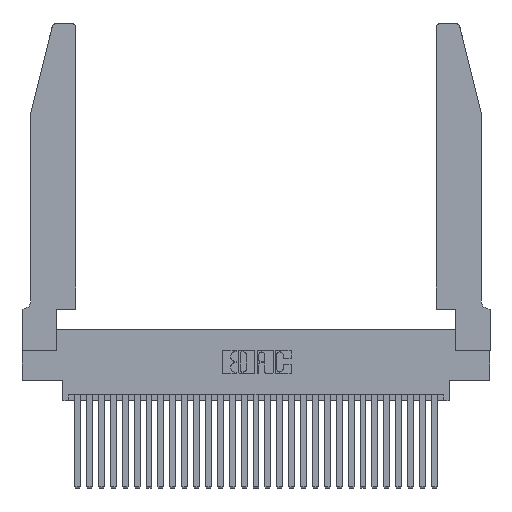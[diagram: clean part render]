
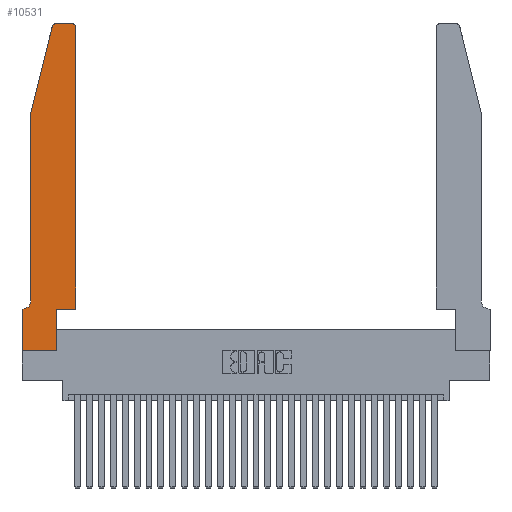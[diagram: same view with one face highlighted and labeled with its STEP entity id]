
A CAD part, top view. The second image highlights one B-rep face of the part: STEP entity #10531.
In plain terms, the highlighted planar face has unit normal (0, 0, 1).
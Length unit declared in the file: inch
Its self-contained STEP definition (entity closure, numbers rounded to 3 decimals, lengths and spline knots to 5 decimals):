
#665 = EDGE_CURVE ( 'NONE', #15499, #2017, #19378, .T. ) ;
#767 = AXIS2_PLACEMENT_3D ( 'NONE', #4609, #9463, #13971 ) ;
#970 = VECTOR ( 'NONE', #5539, 39.37008 ) ;
#1278 = LINE ( 'NONE', #6283, #6064 ) ;
#1909 = VERTEX_POINT ( 'NONE', #15012 ) ;
#2017 = VERTEX_POINT ( 'NONE', #3666 ) ;
#2301 = VERTEX_POINT ( 'NONE', #23953 ) ;
#2540 = LINE ( 'NONE', #5385, #27599 ) ;
#2636 = DIRECTION ( 'NONE',  ( 0., -1., 0. ) ) ;
#2901 = ORIENTED_EDGE ( 'NONE', *, *, #28253, .T. ) ;
#3137 = CARTESIAN_POINT ( 'NONE',  ( 0.4205, 2.75, 0.37 ) ) ;
#3196 = DIRECTION ( 'NONE',  ( 0., 0., -1. ) ) ;
#3589 = ORIENTED_EDGE ( 'NONE', *, *, #21589, .T. ) ;
#3666 = CARTESIAN_POINT ( 'NONE',  ( 0.2865, 0.35, 0.37 ) ) ;
#3855 = VECTOR ( 'NONE', #19013, 39.37008 ) ;
#4079 = PLANE ( 'NONE',  #22951 ) ;
#4118 = ORIENTED_EDGE ( 'NONE', *, *, #4753, .T. ) ;
#4363 = ORIENTED_EDGE ( 'NONE', *, *, #16770, .T. ) ;
#4410 = VECTOR ( 'NONE', #2636, 39.37008 ) ;
#4609 = CARTESIAN_POINT ( 'NONE',  ( 0.284, 2.72, 0.37 ) ) ;
#4753 = EDGE_CURVE ( 'NONE', #11887, #10469, #20247, .T. ) ;
#5385 = CARTESIAN_POINT ( 'NONE',  ( 0., 0., 0.37 ) ) ;
#5526 = EDGE_CURVE ( 'NONE', #10469, #15499, #2540, .T. ) ;
#5539 = DIRECTION ( 'NONE',  ( 0., 1., 0. ) ) ;
#6064 = VECTOR ( 'NONE', #11337, 39.37008 ) ;
#6231 = DIRECTION ( 'NONE',  ( 1., 0., 0. ) ) ;
#6283 = CARTESIAN_POINT ( 'NONE',  ( 0.4505, 0.35, 0.37 ) ) ;
#6318 = DIRECTION ( 'NONE',  ( 1., 0., 0. ) ) ;
#6626 = DIRECTION ( 'NONE',  ( 1., 0., 0. ) ) ;
#6947 = VECTOR ( 'NONE', #21831, 39.37008 ) ;
#7216 = CARTESIAN_POINT ( 'NONE',  ( 0.25487, 2.72718, 0.37 ) ) ;
#7850 = LINE ( 'NONE', #22878, #19965 ) ;
#8911 = ORIENTED_EDGE ( 'NONE', *, *, #27764, .T. ) ;
#9463 = DIRECTION ( 'NONE',  ( 0., 0., 1. ) ) ;
#9594 = VERTEX_POINT ( 'NONE', #7216 ) ;
#10469 = VERTEX_POINT ( 'NONE', #22203 ) ;
#10531 = ADVANCED_FACE ( 'NONE', ( #23017 ), #4079, .T. ) ;
#11265 = CARTESIAN_POINT ( 'NONE',  ( 0.4205, 2.72, 0.37 ) ) ;
#11337 = DIRECTION ( 'NONE',  ( 0., 1., 0. ) ) ;
#11369 = DIRECTION ( 'NONE',  ( 0., 0., 1. ) ) ;
#11523 = VECTOR ( 'NONE', #6626, 39.37008 ) ;
#11709 = CARTESIAN_POINT ( 'NONE',  ( 0.4505, 2.72, 0.37 ) ) ;
#11887 = VERTEX_POINT ( 'NONE', #18778 ) ;
#12079 = CARTESIAN_POINT ( 'NONE',  ( 0.2865, 0., 0.37 ) ) ;
#12588 = CARTESIAN_POINT ( 'NONE',  ( 0.0755, 0.42, 0.37 ) ) ;
#13971 = DIRECTION ( 'NONE',  ( 1., 0., 0. ) ) ;
#15012 = CARTESIAN_POINT ( 'NONE',  ( 0.0755, 2., 0.37 ) ) ;
#15499 = VERTEX_POINT ( 'NONE', #12079 ) ;
#15809 = CIRCLE ( 'NONE', #17748, 0.03 ) ;
#16728 = CARTESIAN_POINT ( 'NONE',  ( 0., 0., 0.37 ) ) ;
#16770 = EDGE_CURVE ( 'NONE', #1909, #19231, #28197, .T. ) ;
#17245 = ORIENTED_EDGE ( 'NONE', *, *, #29105, .T. ) ;
#17280 = CARTESIAN_POINT ( 'NONE',  ( 0.2605, 2.75, 0.37 ) ) ;
#17287 = CARTESIAN_POINT ( 'NONE',  ( 0.0055, 0.42, 0.37 ) ) ;
#17748 = AXIS2_PLACEMENT_3D ( 'NONE', #11265, #11369, #6318 ) ;
#17902 = ORIENTED_EDGE ( 'NONE', *, *, #27622, .T. ) ;
#18322 = ORIENTED_EDGE ( 'NONE', *, *, #30302, .T. ) ;
#18445 = CARTESIAN_POINT ( 'NONE',  ( 0.0055, 0.35, 0.37 ) ) ;
#18459 = EDGE_CURVE ( 'NONE', #28261, #9594, #26662, .T. ) ;
#18778 = CARTESIAN_POINT ( 'NONE',  ( 0., 0.35, 0.37 ) ) ;
#19013 = DIRECTION ( 'NONE',  ( 0., -1., 0. ) ) ;
#19231 = VERTEX_POINT ( 'NONE', #12588 ) ;
#19378 = LINE ( 'NONE', #19747, #970 ) ;
#19660 = DIRECTION ( 'NONE',  ( -1., 0., 0. ) ) ;
#19747 = CARTESIAN_POINT ( 'NONE',  ( 0.2865, 0.35, 0.37 ) ) ;
#19965 = VECTOR ( 'NONE', #26800, 39.37008 ) ;
#20247 = LINE ( 'NONE', #16728, #4410 ) ;
#20531 = EDGE_CURVE ( 'NONE', #22021, #22831, #15809, .T. ) ;
#21589 = EDGE_CURVE ( 'NONE', #22831, #28261, #25352, .T. ) ;
#21831 = DIRECTION ( 'NONE',  ( -1., 0., 0. ) ) ;
#22021 = VERTEX_POINT ( 'NONE', #11709 ) ;
#22048 = CARTESIAN_POINT ( 'NONE',  ( 0.284, 2.75, 0.37 ) ) ;
#22203 = CARTESIAN_POINT ( 'NONE',  ( 0., 0., 0.37 ) ) ;
#22426 = ORIENTED_EDGE ( 'NONE', *, *, #20531, .T. ) ;
#22434 = ORIENTED_EDGE ( 'NONE', *, *, #5526, .T. ) ;
#22638 = CIRCLE ( 'NONE', #29342, 0.07 ) ;
#22831 = VERTEX_POINT ( 'NONE', #3137 ) ;
#22878 = CARTESIAN_POINT ( 'NONE',  ( 0.0755, 2., 0.37 ) ) ;
#22951 = AXIS2_PLACEMENT_3D ( 'NONE', #27673, #30051, #6231 ) ;
#23017 = FACE_OUTER_BOUND ( 'NONE', #23213, .T. ) ;
#23213 = EDGE_LOOP ( 'NONE', ( #3589, #27527, #18322, #4363, #2901, #17902, #4118, #22434, #28349, #17245, #8911, #22426 ) ) ;
#23953 = CARTESIAN_POINT ( 'NONE',  ( 0.4505, 0.35, 0.37 ) ) ;
#23964 = VERTEX_POINT ( 'NONE', #18445 ) ;
#24739 = DIRECTION ( 'NONE',  ( -1., 0., 0. ) ) ;
#25352 = LINE ( 'NONE', #17280, #6947 ) ;
#25517 = LINE ( 'NONE', #25678, #11523 ) ;
#25678 = CARTESIAN_POINT ( 'NONE',  ( 0.4505, 0.35, 0.37 ) ) ;
#25719 = CARTESIAN_POINT ( 'NONE',  ( 0.0755, 2., 0.37 ) ) ;
#26364 = VECTOR ( 'NONE', #24739, 39.37008 ) ;
#26662 = CIRCLE ( 'NONE', #767, 0.03 ) ;
#26800 = DIRECTION ( 'NONE',  ( -0.239, -0.971, 0. ) ) ;
#27527 = ORIENTED_EDGE ( 'NONE', *, *, #18459, .T. ) ;
#27599 = VECTOR ( 'NONE', #29090, 39.37008 ) ;
#27622 = EDGE_CURVE ( 'NONE', #23964, #11887, #30435, .T. ) ;
#27673 = CARTESIAN_POINT ( 'NONE',  ( 0., 0.35, 0.37 ) ) ;
#27764 = EDGE_CURVE ( 'NONE', #2301, #22021, #1278, .T. ) ;
#28197 = LINE ( 'NONE', #25719, #3855 ) ;
#28253 = EDGE_CURVE ( 'NONE', #19231, #23964, #22638, .T. ) ;
#28261 = VERTEX_POINT ( 'NONE', #22048 ) ;
#28349 = ORIENTED_EDGE ( 'NONE', *, *, #665, .T. ) ;
#29090 = DIRECTION ( 'NONE',  ( 1., 0., 0. ) ) ;
#29105 = EDGE_CURVE ( 'NONE', #2017, #2301, #25517, .T. ) ;
#29342 = AXIS2_PLACEMENT_3D ( 'NONE', #17287, #3196, #19660 ) ;
#29499 = CARTESIAN_POINT ( 'NONE',  ( 0.0755, 0.35, 0.37 ) ) ;
#30051 = DIRECTION ( 'NONE',  ( 0., 0., 1. ) ) ;
#30302 = EDGE_CURVE ( 'NONE', #9594, #1909, #7850, .T. ) ;
#30435 = LINE ( 'NONE', #29499, #26364 ) ;
